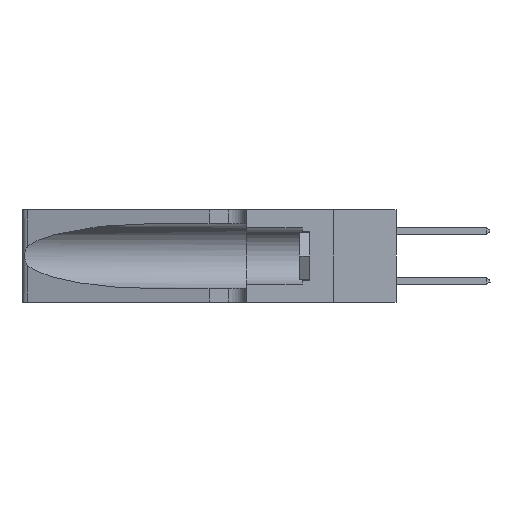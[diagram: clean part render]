
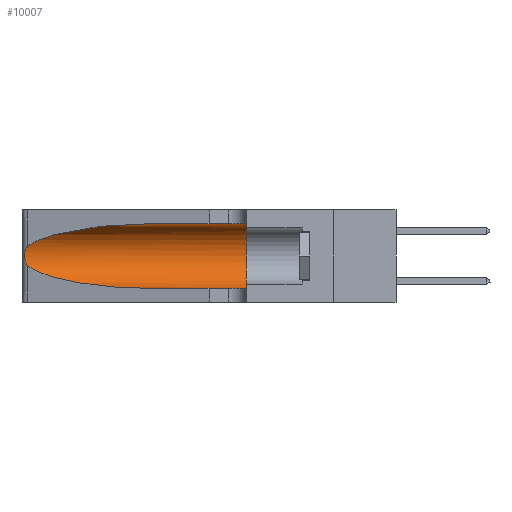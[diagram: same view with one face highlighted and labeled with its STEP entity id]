
A CAD part, left-side view. The second image highlights one B-rep face of the part: STEP entity #10007.
In plain terms, the highlighted cylindrical face has radius 3.308 mm (diameter 6.617 mm), a partial arc.
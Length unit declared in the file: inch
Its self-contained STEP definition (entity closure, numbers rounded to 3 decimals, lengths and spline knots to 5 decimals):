
#634 = VERTEX_POINT ( 'NONE', #29777 ) ;
#1129 = EDGE_CURVE ( 'NONE', #25228, #27982, #26750, .T. ) ;
#1557 = DIRECTION ( 'NONE',  ( 0., -1., 0. ) ) ;
#2138 = CARTESIAN_POINT ( 'NONE',  ( 0.26018, 1.23835, 0.19895 ) ) ;
#2197 = AXIS2_PLACEMENT_3D ( 'NONE', #20395, #1557, #4463 ) ;
#2252 = CARTESIAN_POINT ( 'NONE',  ( 0.25487, 1.22718, 0.14631 ) ) ;
#2466 = CARTESIAN_POINT ( 'NONE',  ( 0.25854, 1.2359, 0.20912 ) ) ;
#2806 = VERTEX_POINT ( 'NONE', #33648 ) ;
#3969 = EDGE_CURVE ( 'NONE', #27982, #15187, #20745, .T. ) ;
#4463 = DIRECTION ( 'NONE',  ( 0., 0., -1. ) ) ;
#5104 = CARTESIAN_POINT ( 'NONE',  ( 0.25555, 1.22994, 0.2215 ) ) ;
#5570 = CARTESIAN_POINT ( 'NONE',  ( 0.25487, 1.22718, 0.14631 ) ) ;
#5884 = VECTOR ( 'NONE', #17144, 39.37008 ) ;
#7387 = ORIENTED_EDGE ( 'NONE', *, *, #33009, .T. ) ;
#7640 = CARTESIAN_POINT ( 'NONE',  ( 0.26075, 1.23896, 0.19203 ) ) ;
#9000 = CARTESIAN_POINT ( 'NONE',  ( 0.1305, 1.61858, 0.31525 ) ) ;
#9479 = CARTESIAN_POINT ( 'NONE',  ( 0.1305, 0.35, 0.185 ) ) ;
#10007 = ADVANCED_FACE ( 'NONE', ( #13900 ), #31148, .F. ) ;
#10161 = CARTESIAN_POINT ( 'NONE',  ( 0.26017, 1.23833, 0.17102 ) ) ;
#10353 = CARTESIAN_POINT ( 'NONE',  ( 0.18966, 0.96281, 0.31525 ) ) ;
#10380 = CARTESIAN_POINT ( 'NONE',  ( 0.25856, 1.23593, 0.16098 ) ) ;
#10861 = LINE ( 'NONE', #9000, #5884 ) ;
#11587 = VERTEX_POINT ( 'NONE', #14810 ) ;
#11855 = DIRECTION ( 'NONE',  ( 0., 1., 0. ) ) ;
#12185 = CARTESIAN_POINT ( 'NONE',  ( 0.25487, 1.22718, 0.14631 ) ) ;
#12544 = ORIENTED_EDGE ( 'NONE', *, *, #3969, .T. ) ;
#12662 = CARTESIAN_POINT ( 'NONE',  ( 0.18966, 0.96281, 0.05475 ) ) ;
#12892 = CARTESIAN_POINT ( 'NONE',  ( 0.25789, 1.23486, 0.15765 ) ) ;
#13649 = EDGE_CURVE ( 'NONE', #634, #2806, #27616, .T. ) ;
#13688 = CARTESIAN_POINT ( 'NONE',  ( 0.1305, 0.72297, 0.05475 ) ) ;
#13900 = FACE_OUTER_BOUND ( 'NONE', #32421, .T. ) ;
#14235 = DIRECTION ( 'NONE',  ( 0., 0., 1. ) ) ;
#14443 = CARTESIAN_POINT ( 'NONE',  ( 0.1305, 1.61858, 0.05475 ) ) ;
#14810 = CARTESIAN_POINT ( 'NONE',  ( 0.1305, 0.72297, 0.31525 ) ) ;
#15187 = VERTEX_POINT ( 'NONE', #22492 ) ;
#15327 = CARTESIAN_POINT ( 'NONE',  ( 0.26075, 1.23896, 0.178 ) ) ;
#15431 = CARTESIAN_POINT ( 'NONE',  ( 0.25487, 1.22718, 0.22369 ) ) ;
#15655 = AXIS2_PLACEMENT_3D ( 'NONE', #9479, #11855, #14235 ) ;
#16028 = ORIENTED_EDGE ( 'NONE', *, *, #26642, .F. ) ;
#16293 = CARTESIAN_POINT ( 'NONE',  ( 0.25487, 1.22718, 0.22369 ) ) ;
#17144 = DIRECTION ( 'NONE',  ( 0., -1., 0. ) ) ;
#19336 = ORIENTED_EDGE ( 'NONE', *, *, #19830, .T. ) ;
#19830 = EDGE_CURVE ( 'NONE', #15187, #2806, #29766, .T. ) ;
#20315 =( BOUNDED_CURVE ( )  B_SPLINE_CURVE ( 3, ( #33643, #10353, #33743, #20552 ),
 .UNSPECIFIED., .F., .T. ) 
 B_SPLINE_CURVE_WITH_KNOTS ( ( 4, 4 ),
 ( 1.5708, 2.84003 ),
 .UNSPECIFIED. ) 
 CURVE ( )  GEOMETRIC_REPRESENTATION_ITEM ( )  RATIONAL_B_SPLINE_CURVE ( ( 1., 0.87, 0.87, 1. ) ) 
 REPRESENTATION_ITEM ( '' )  );
#20395 = CARTESIAN_POINT ( 'NONE',  ( 0.1305, 1.61858, 0.185 ) ) ;
#20552 = CARTESIAN_POINT ( 'NONE',  ( 0.25487, 1.22718, 0.22369 ) ) ;
#20745 =( BOUNDED_CURVE ( )  B_SPLINE_CURVE ( 3, ( #12185, #31756, #12662, #13688 ),
 .UNSPECIFIED., .F., .F. ) 
 B_SPLINE_CURVE_WITH_KNOTS ( ( 4, 4 ),
 ( 3.44316, 4.71239 ),
 .UNSPECIFIED. ) 
 CURVE ( )  GEOMETRIC_REPRESENTATION_ITEM ( )  RATIONAL_B_SPLINE_CURVE ( ( 1., 0.87, 0.87, 1. ) ) 
 REPRESENTATION_ITEM ( '' )  );
#22014 = DIRECTION ( 'NONE',  ( 0., -1., 0. ) ) ;
#22492 = CARTESIAN_POINT ( 'NONE',  ( 0.1305, 0.72297, 0.05475 ) ) ;
#22944 = VECTOR ( 'NONE', #22014, 39.37008 ) ;
#23223 = CARTESIAN_POINT ( 'NONE',  ( 0.25639, 1.23184, 0.21858 ) ) ;
#25228 = VERTEX_POINT ( 'NONE', #16293 ) ;
#26642 = EDGE_CURVE ( 'NONE', #11587, #634, #10861, .T. ) ;
#26750 = B_SPLINE_CURVE_WITH_KNOTS ( 'NONE', 3,
 ( #15431, #5104, #23223, #28324, #2466, #2138, #7640, #15327, #10161, #10380, #12892, #33560, #31164, #2252 ),
 .UNSPECIFIED., .F., .F.,
 ( 4, 2, 2, 2, 2, 2, 4 ),
 ( 0., 0.00027, 0.00053, 0.00107, 0.0016, 0.00187, 0.00214 ),
 .UNSPECIFIED. ) ;
#27616 = CIRCLE ( 'NONE', #15655, 0.13025 ) ;
#27982 = VERTEX_POINT ( 'NONE', #5570 ) ;
#28324 = CARTESIAN_POINT ( 'NONE',  ( 0.25787, 1.23484, 0.2124 ) ) ;
#29766 = LINE ( 'NONE', #14443, #22944 ) ;
#29777 = CARTESIAN_POINT ( 'NONE',  ( 0.1305, 0.35, 0.31525 ) ) ;
#30289 = ORIENTED_EDGE ( 'NONE', *, *, #13649, .F. ) ;
#31148 = CYLINDRICAL_SURFACE ( 'NONE', #2197, 0.13025 ) ;
#31164 = CARTESIAN_POINT ( 'NONE',  ( 0.25555, 1.22993, 0.14849 ) ) ;
#31756 = CARTESIAN_POINT ( 'NONE',  ( 0.2373, 1.15595, 0.08982 ) ) ;
#31838 = ORIENTED_EDGE ( 'NONE', *, *, #1129, .T. ) ;
#32421 = EDGE_LOOP ( 'NONE', ( #7387, #31838, #12544, #19336, #30289, #16028 ) ) ;
#33009 = EDGE_CURVE ( 'NONE', #11587, #25228, #20315, .T. ) ;
#33560 = CARTESIAN_POINT ( 'NONE',  ( 0.25639, 1.23186, 0.15144 ) ) ;
#33643 = CARTESIAN_POINT ( 'NONE',  ( 0.1305, 0.72297, 0.31525 ) ) ;
#33648 = CARTESIAN_POINT ( 'NONE',  ( 0.1305, 0.35, 0.05475 ) ) ;
#33743 = CARTESIAN_POINT ( 'NONE',  ( 0.2373, 1.15595, 0.28018 ) ) ;
